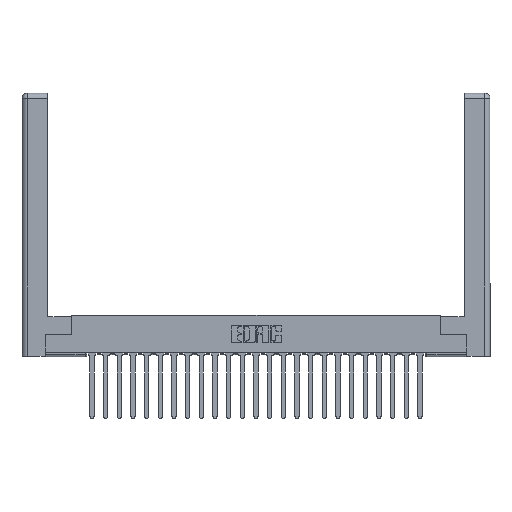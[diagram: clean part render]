
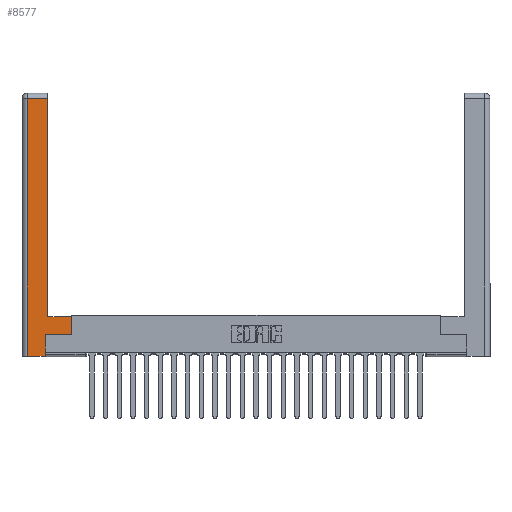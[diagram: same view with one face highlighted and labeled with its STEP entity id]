
A CAD part, top view. The second image highlights one B-rep face of the part: STEP entity #8577.
In plain terms, the highlighted planar face has unit normal (0, 0, 1).
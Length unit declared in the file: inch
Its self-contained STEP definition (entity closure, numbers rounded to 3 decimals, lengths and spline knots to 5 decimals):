
#196 = ORIENTED_EDGE ( 'NONE', *, *, #19766, .T. ) ;
#391 = VERTEX_POINT ( 'NONE', #5455 ) ;
#478 = FACE_OUTER_BOUND ( 'NONE', #1687, .T. ) ;
#608 = AXIS2_PLACEMENT_3D ( 'NONE', #12371, #6684, #18332 ) ;
#761 = VECTOR ( 'NONE', #1241, 39.37008 ) ;
#979 = CARTESIAN_POINT ( 'NONE',  ( 0.265, 0.245, 0. ) ) ;
#1241 = DIRECTION ( 'NONE',  ( 0., 1., 0. ) ) ;
#1567 = VERTEX_POINT ( 'NONE', #7662 ) ;
#1675 = EDGE_CURVE ( 'NONE', #12744, #19595, #6954, .T. ) ;
#1687 = EDGE_LOOP ( 'NONE', ( #3582, #6941, #22558, #20365, #196, #24527, #3574, #8529 ) ) ;
#1749 = LINE ( 'NONE', #9802, #17329 ) ;
#2155 = CARTESIAN_POINT ( 'NONE',  ( 0.565, 0.245, 0. ) ) ;
#2391 = LINE ( 'NONE', #20508, #10926 ) ;
#2887 = LINE ( 'NONE', #14922, #8305 ) ;
#3574 = ORIENTED_EDGE ( 'NONE', *, *, #17450, .T. ) ;
#3582 = ORIENTED_EDGE ( 'NONE', *, *, #15162, .T. ) ;
#5119 = CARTESIAN_POINT ( 'NONE',  ( 0.295, 0.45, 0. ) ) ;
#5207 = LINE ( 'NONE', #979, #761 ) ;
#5455 = CARTESIAN_POINT ( 'NONE',  ( 0.265, 0., 0. ) ) ;
#6101 = DIRECTION ( 'NONE',  ( 0., -1., 0. ) ) ;
#6374 = LINE ( 'NONE', #14431, #24948 ) ;
#6684 = DIRECTION ( 'NONE',  ( 0., 0., -1. ) ) ;
#6685 = VERTEX_POINT ( 'NONE', #25905 ) ;
#6728 = DIRECTION ( 'NONE',  ( -1., 0., 0. ) ) ;
#6941 = ORIENTED_EDGE ( 'NONE', *, *, #18784, .T. ) ;
#6954 = LINE ( 'NONE', #5119, #7460 ) ;
#7460 = VECTOR ( 'NONE', #12907, 39.37008 ) ;
#7662 = CARTESIAN_POINT ( 'NONE',  ( 0.0615, 2.94, 0. ) ) ;
#7672 = VERTEX_POINT ( 'NONE', #2155 ) ;
#8305 = VECTOR ( 'NONE', #6728, 39.37008 ) ;
#8396 = LINE ( 'NONE', #14224, #18994 ) ;
#8529 = ORIENTED_EDGE ( 'NONE', *, *, #1675, .T. ) ;
#8577 = ADVANCED_FACE ( 'NONE', ( #478 ), #20577, .F. ) ;
#9369 = CARTESIAN_POINT ( 'NONE',  ( 0.295, 2.94, 0. ) ) ;
#9802 = CARTESIAN_POINT ( 'NONE',  ( 0.565, 0.45, 0. ) ) ;
#9970 = CARTESIAN_POINT ( 'NONE',  ( 0.265, 0., 0. ) ) ;
#10926 = VECTOR ( 'NONE', #14683, 39.37008 ) ;
#11835 = DIRECTION ( 'NONE',  ( 1., 0., 0. ) ) ;
#12371 = CARTESIAN_POINT ( 'NONE',  ( 0., 0., 0. ) ) ;
#12611 = CARTESIAN_POINT ( 'NONE',  ( 0.0615, 0., 0. ) ) ;
#12744 = VERTEX_POINT ( 'NONE', #20574 ) ;
#12907 = DIRECTION ( 'NONE',  ( -1., 0., 0. ) ) ;
#14224 = CARTESIAN_POINT ( 'NONE',  ( 0.295, 3., 0. ) ) ;
#14417 = EDGE_CURVE ( 'NONE', #6685, #7672, #2391, .T. ) ;
#14431 = CARTESIAN_POINT ( 'NONE',  ( 0.0615, 0., 0. ) ) ;
#14615 = VERTEX_POINT ( 'NONE', #9369 ) ;
#14683 = DIRECTION ( 'NONE',  ( 1., 0., 0. ) ) ;
#14922 = CARTESIAN_POINT ( 'NONE',  ( 0.0615, 2.94, 0. ) ) ;
#15162 = EDGE_CURVE ( 'NONE', #19595, #14615, #8396, .T. ) ;
#16325 = CARTESIAN_POINT ( 'NONE',  ( 0.295, 0.45, 0. ) ) ;
#17329 = VECTOR ( 'NONE', #25951, 39.37008 ) ;
#17442 = EDGE_CURVE ( 'NONE', #1567, #25844, #6374, .T. ) ;
#17450 = EDGE_CURVE ( 'NONE', #7672, #12744, #1749, .T. ) ;
#18332 = DIRECTION ( 'NONE',  ( -1., 0., 0. ) ) ;
#18784 = EDGE_CURVE ( 'NONE', #14615, #1567, #2887, .T. ) ;
#18994 = VECTOR ( 'NONE', #20317, 39.37008 ) ;
#19520 = EDGE_CURVE ( 'NONE', #25844, #391, #23860, .T. ) ;
#19595 = VERTEX_POINT ( 'NONE', #16325 ) ;
#19766 = EDGE_CURVE ( 'NONE', #391, #6685, #5207, .T. ) ;
#20317 = DIRECTION ( 'NONE',  ( 0., 1., 0. ) ) ;
#20365 = ORIENTED_EDGE ( 'NONE', *, *, #19520, .T. ) ;
#20508 = CARTESIAN_POINT ( 'NONE',  ( 0.565, 0.245, 0. ) ) ;
#20574 = CARTESIAN_POINT ( 'NONE',  ( 0.565, 0.45, 0. ) ) ;
#20577 = PLANE ( 'NONE',  #608 ) ;
#22558 = ORIENTED_EDGE ( 'NONE', *, *, #17442, .T. ) ;
#23860 = LINE ( 'NONE', #9970, #25646 ) ;
#24527 = ORIENTED_EDGE ( 'NONE', *, *, #14417, .T. ) ;
#24948 = VECTOR ( 'NONE', #6101, 39.37008 ) ;
#25646 = VECTOR ( 'NONE', #11835, 39.37008 ) ;
#25844 = VERTEX_POINT ( 'NONE', #12611 ) ;
#25905 = CARTESIAN_POINT ( 'NONE',  ( 0.265, 0.245, 0. ) ) ;
#25951 = DIRECTION ( 'NONE',  ( 0., 1., 0. ) ) ;
